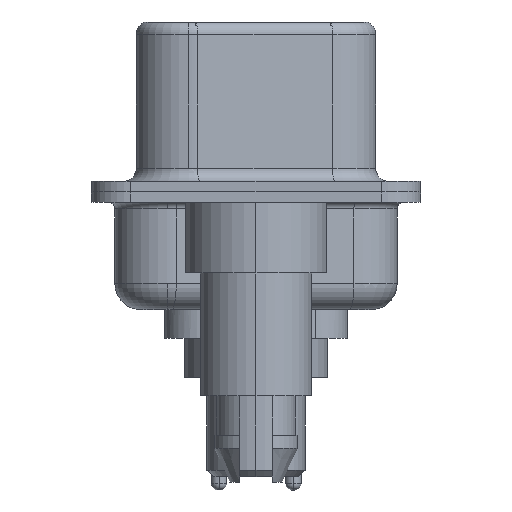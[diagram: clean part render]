
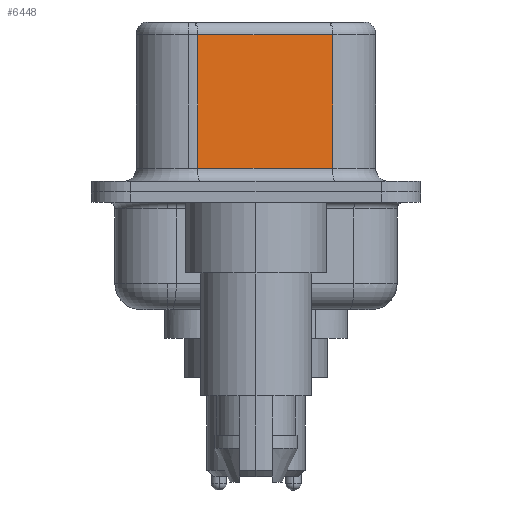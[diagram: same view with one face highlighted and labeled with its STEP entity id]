
A CAD part, left-side view. The second image highlights one B-rep face of the part: STEP entity #6448.
In plain terms, the highlighted planar face has unit normal (-0.985, -0.174, 0).
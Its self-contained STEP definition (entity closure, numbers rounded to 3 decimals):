
#157 = CARTESIAN_POINT ( 'NONE',  ( 4.58, -2.927, 6.52 ) ) ;
#510 = EDGE_CURVE ( 'NONE', #11470, #20661, #16311, .T. ) ;
#710 = ORIENTED_EDGE ( 'NONE', *, *, #19436, .F. ) ;
#1362 = PLANE ( 'NONE',  #18032 ) ;
#1452 = CARTESIAN_POINT ( 'NONE',  ( 4.58, -2.927, 6.52 ) ) ;
#1567 = DIRECTION ( 'NONE',  ( 0.985, 0.174, 0. ) ) ;
#3188 = CARTESIAN_POINT ( 'NONE',  ( 4.58, -2.927, 0.9 ) ) ;
#5834 = EDGE_LOOP ( 'NONE', ( #710, #21067, #21463, #7155 ) ) ;
#6138 = DIRECTION ( 'NONE',  ( 0., 0., -1. ) ) ;
#6183 = VECTOR ( 'NONE', #22072, 1000. ) ;
#6254 = CARTESIAN_POINT ( 'NONE',  ( 3.67, 2.233, 6.02 ) ) ;
#6448 = ADVANCED_FACE ( 'NONE', ( #22686 ), #1362, .F. ) ;
#7155 = ORIENTED_EDGE ( 'NONE', *, *, #10296, .T. ) ;
#8332 = VERTEX_POINT ( 'NONE', #3188 ) ;
#9755 = CARTESIAN_POINT ( 'NONE',  ( 4.58, -2.927, 6.02 ) ) ;
#10296 = EDGE_CURVE ( 'NONE', #20401, #8332, #21511, .T. ) ;
#10483 = VECTOR ( 'NONE', #27689, 1000. ) ;
#11470 = VERTEX_POINT ( 'NONE', #9755 ) ;
#14839 = CARTESIAN_POINT ( 'NONE',  ( 3.67, 2.233, 6.52 ) ) ;
#15039 = DIRECTION ( 'NONE',  ( -0.174, 0.985, 0. ) ) ;
#15244 = EDGE_CURVE ( 'NONE', #20661, #20401, #21812, .T. ) ;
#15701 = VECTOR ( 'NONE', #16437, 1000. ) ;
#16311 = LINE ( 'NONE', #27341, #10483 ) ;
#16437 = DIRECTION ( 'NONE',  ( 0.174, -0.985, 0. ) ) ;
#18032 = AXIS2_PLACEMENT_3D ( 'NONE', #1452, #1567, #15039 ) ;
#18078 = VECTOR ( 'NONE', #6138, 1000. ) ;
#18529 = LINE ( 'NONE', #157, #6183 ) ;
#19436 = EDGE_CURVE ( 'NONE', #11470, #8332, #18529, .T. ) ;
#20401 = VERTEX_POINT ( 'NONE', #23018 ) ;
#20661 = VERTEX_POINT ( 'NONE', #6254 ) ;
#21067 = ORIENTED_EDGE ( 'NONE', *, *, #510, .T. ) ;
#21463 = ORIENTED_EDGE ( 'NONE', *, *, #15244, .T. ) ;
#21511 = LINE ( 'NONE', #27304, #15701 ) ;
#21812 = LINE ( 'NONE', #14839, #18078 ) ;
#22072 = DIRECTION ( 'NONE',  ( 0., 0., -1. ) ) ;
#22686 = FACE_OUTER_BOUND ( 'NONE', #5834, .T. ) ;
#23018 = CARTESIAN_POINT ( 'NONE',  ( 3.67, 2.233, 0.9 ) ) ;
#27304 = CARTESIAN_POINT ( 'NONE',  ( 4.58, -2.927, 0.9 ) ) ;
#27341 = CARTESIAN_POINT ( 'NONE',  ( 4.58, -2.927, 6.02 ) ) ;
#27689 = DIRECTION ( 'NONE',  ( -0.174, 0.985, 0. ) ) ;
